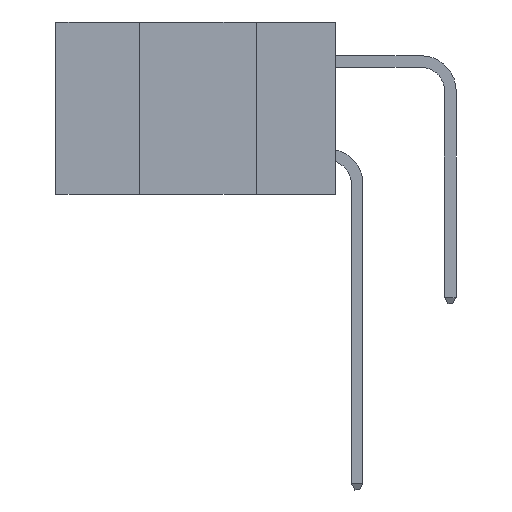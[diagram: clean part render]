
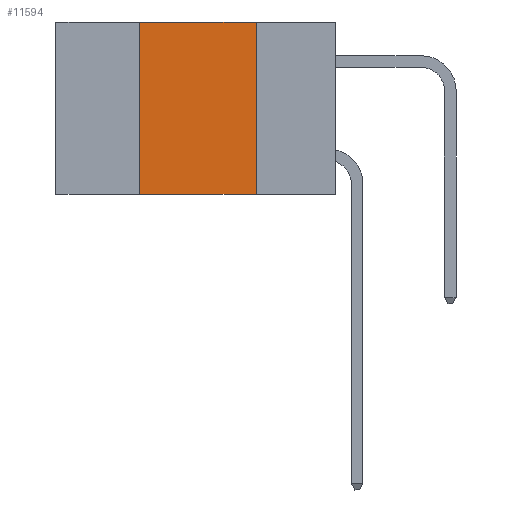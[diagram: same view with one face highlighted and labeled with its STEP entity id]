
A CAD part, left-side view. The second image highlights one B-rep face of the part: STEP entity #11594.
In plain terms, the highlighted planar face has unit normal (-1, 0, 0).
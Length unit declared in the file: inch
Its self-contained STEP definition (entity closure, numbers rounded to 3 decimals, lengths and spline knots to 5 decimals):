
#295 = VERTEX_POINT ( 'NONE', #12579 ) ;
#411 = ORIENTED_EDGE ( 'NONE', *, *, #14796, .F. ) ;
#594 = LINE ( 'NONE', #7773, #12521 ) ;
#975 = VECTOR ( 'NONE', #16263, 39.37008 ) ;
#1141 = CARTESIAN_POINT ( 'NONE',  ( 0., 0.17, 0. ) ) ;
#2001 = VERTEX_POINT ( 'NONE', #1141 ) ;
#2161 = CARTESIAN_POINT ( 'NONE',  ( 0., 0.42, 0. ) ) ;
#2286 = PLANE ( 'NONE',  #14432 ) ;
#2346 = CARTESIAN_POINT ( 'NONE',  ( 0., 0.42, 0. ) ) ;
#2757 = DIRECTION ( 'NONE',  ( 0., 0., -1. ) ) ;
#3008 = DIRECTION ( 'NONE',  ( 0., -1., 0. ) ) ;
#3393 = ORIENTED_EDGE ( 'NONE', *, *, #8364, .F. ) ;
#4355 = EDGE_CURVE ( 'NONE', #295, #8365, #594, .T. ) ;
#5823 = VERTEX_POINT ( 'NONE', #2161 ) ;
#6162 = LINE ( 'NONE', #11230, #975 ) ;
#6481 = DIRECTION ( 'NONE',  ( 1., 0., 0. ) ) ;
#7349 = EDGE_CURVE ( 'NONE', #295, #5823, #7382, .T. ) ;
#7382 = LINE ( 'NONE', #2346, #7534 ) ;
#7534 = VECTOR ( 'NONE', #8624, 39.37008 ) ;
#7773 = CARTESIAN_POINT ( 'NONE',  ( 0., 0.6, -0.37 ) ) ;
#8364 = EDGE_CURVE ( 'NONE', #2001, #8365, #6162, .T. ) ;
#8365 = VERTEX_POINT ( 'NONE', #9975 ) ;
#8471 = VECTOR ( 'NONE', #3008, 39.37008 ) ;
#8624 = DIRECTION ( 'NONE',  ( 0., 0., 1. ) ) ;
#9208 = CARTESIAN_POINT ( 'NONE',  ( 0., 0.6, 0. ) ) ;
#9975 = CARTESIAN_POINT ( 'NONE',  ( 0., 0.17, -0.37 ) ) ;
#10348 = DIRECTION ( 'NONE',  ( 0., -1., 0. ) ) ;
#10462 = CARTESIAN_POINT ( 'NONE',  ( 0., 0.6, 0. ) ) ;
#10542 = LINE ( 'NONE', #9208, #8471 ) ;
#11230 = CARTESIAN_POINT ( 'NONE',  ( 0., 0.17, 0. ) ) ;
#11594 = ADVANCED_FACE ( 'NONE', ( #13610 ), #2286, .F. ) ;
#12521 = VECTOR ( 'NONE', #10348, 39.37008 ) ;
#12579 = CARTESIAN_POINT ( 'NONE',  ( 0., 0.42, -0.37 ) ) ;
#13610 = FACE_OUTER_BOUND ( 'NONE', #15082, .T. ) ;
#13819 = ORIENTED_EDGE ( 'NONE', *, *, #4355, .T. ) ;
#14334 = ORIENTED_EDGE ( 'NONE', *, *, #7349, .F. ) ;
#14432 = AXIS2_PLACEMENT_3D ( 'NONE', #10462, #6481, #2757 ) ;
#14796 = EDGE_CURVE ( 'NONE', #5823, #2001, #10542, .T. ) ;
#15082 = EDGE_LOOP ( 'NONE', ( #3393, #411, #14334, #13819 ) ) ;
#16263 = DIRECTION ( 'NONE',  ( 0., 0., -1. ) ) ;
